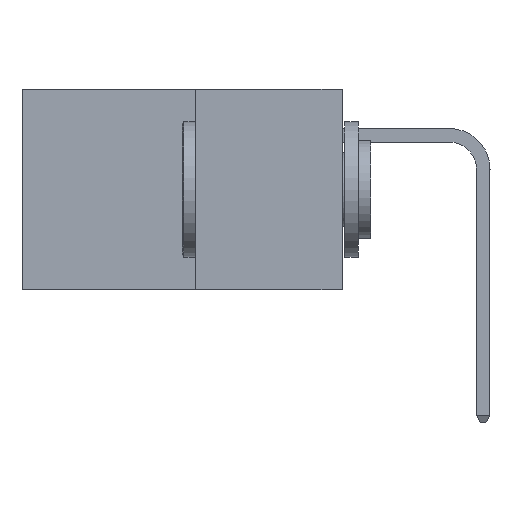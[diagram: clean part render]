
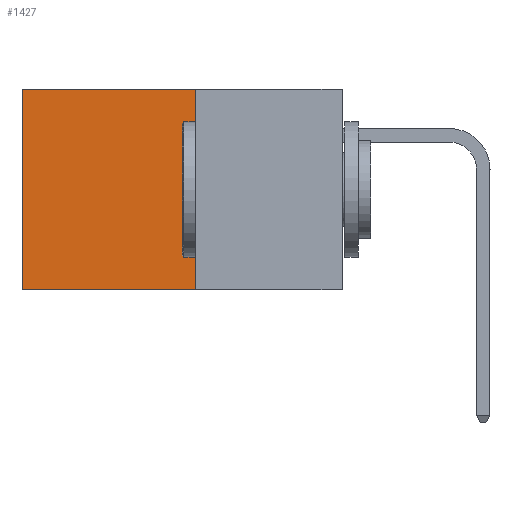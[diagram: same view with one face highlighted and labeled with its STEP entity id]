
A CAD part, left-side view. The second image highlights one B-rep face of the part: STEP entity #1427.
In plain terms, the highlighted planar face has unit normal (-1, 0, 0).
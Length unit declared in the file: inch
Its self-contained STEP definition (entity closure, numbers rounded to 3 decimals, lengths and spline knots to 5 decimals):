
#946 = EDGE_LOOP ( 'NONE', ( #6713, #12769, #7743, #2530 ) ) ;
#1427 = ADVANCED_FACE ( 'NONE', ( #13640 ), #13237, .F. ) ;
#2474 = CARTESIAN_POINT ( 'NONE',  ( 0.277, 0.27, 0. ) ) ;
#2530 = ORIENTED_EDGE ( 'NONE', *, *, #10147, .T. ) ;
#2828 = EDGE_CURVE ( 'NONE', #2933, #7029, #3659, .T. ) ;
#2932 = DIRECTION ( 'NONE',  ( 0., 0., -1. ) ) ;
#2933 = VERTEX_POINT ( 'NONE', #7539 ) ;
#2989 = CARTESIAN_POINT ( 'NONE',  ( 0.277, 0.27, -0.37 ) ) ;
#3299 = VECTOR ( 'NONE', #10943, 39.37008 ) ;
#3659 = LINE ( 'NONE', #11078, #3299 ) ;
#4636 = CARTESIAN_POINT ( 'NONE',  ( 0.277, 0.59, -0.37 ) ) ;
#4861 = CARTESIAN_POINT ( 'NONE',  ( 0.277, 0.27, 0. ) ) ;
#5831 = VERTEX_POINT ( 'NONE', #4861 ) ;
#6713 = ORIENTED_EDGE ( 'NONE', *, *, #11569, .T. ) ;
#7029 = VERTEX_POINT ( 'NONE', #4636 ) ;
#7286 = CARTESIAN_POINT ( 'NONE',  ( 0.277, 0.27, -0.37 ) ) ;
#7379 = VECTOR ( 'NONE', #9069, 39.37008 ) ;
#7539 = CARTESIAN_POINT ( 'NONE',  ( 0.277, 0.27, -0.37 ) ) ;
#7743 = ORIENTED_EDGE ( 'NONE', *, *, #12573, .F. ) ;
#8510 = CARTESIAN_POINT ( 'NONE',  ( 0.277, 0.59, 0. ) ) ;
#9069 = DIRECTION ( 'NONE',  ( 0., 1., 0. ) ) ;
#9274 = VERTEX_POINT ( 'NONE', #8510 ) ;
#9347 = LINE ( 'NONE', #2989, #11852 ) ;
#9589 = DIRECTION ( 'NONE',  ( 0., 0., -1. ) ) ;
#10087 = CARTESIAN_POINT ( 'NONE',  ( 0.277, 0.59, -0.37 ) ) ;
#10147 = EDGE_CURVE ( 'NONE', #5831, #9274, #10599, .T. ) ;
#10557 = AXIS2_PLACEMENT_3D ( 'NONE', #7286, #13062, #2932 ) ;
#10599 = LINE ( 'NONE', #2474, #7379 ) ;
#10943 = DIRECTION ( 'NONE',  ( 0., 1., 0. ) ) ;
#11078 = CARTESIAN_POINT ( 'NONE',  ( 0.277, 0.27, -0.37 ) ) ;
#11168 = DIRECTION ( 'NONE',  ( 0., 0., -1. ) ) ;
#11569 = EDGE_CURVE ( 'NONE', #9274, #7029, #11724, .T. ) ;
#11724 = LINE ( 'NONE', #10087, #14123 ) ;
#11852 = VECTOR ( 'NONE', #9589, 39.37008 ) ;
#12573 = EDGE_CURVE ( 'NONE', #5831, #2933, #9347, .T. ) ;
#12769 = ORIENTED_EDGE ( 'NONE', *, *, #2828, .F. ) ;
#13062 = DIRECTION ( 'NONE',  ( 1., 0., 0. ) ) ;
#13237 = PLANE ( 'NONE',  #10557 ) ;
#13640 = FACE_OUTER_BOUND ( 'NONE', #946, .T. ) ;
#14123 = VECTOR ( 'NONE', #11168, 39.37008 ) ;
